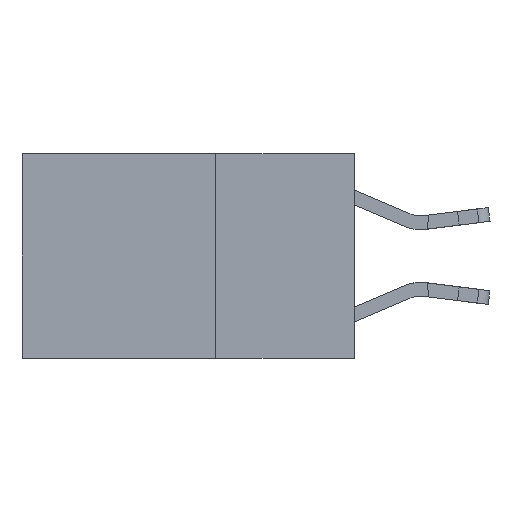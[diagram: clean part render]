
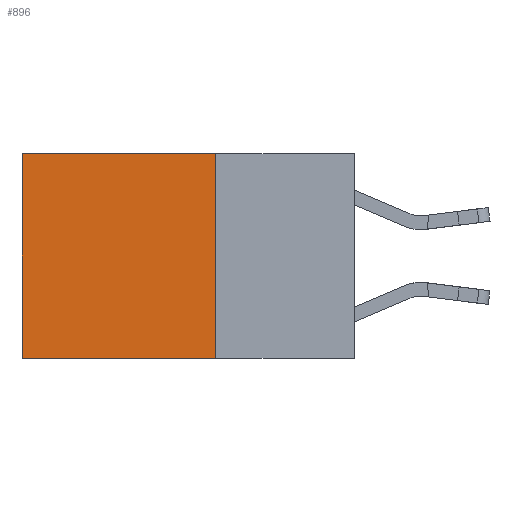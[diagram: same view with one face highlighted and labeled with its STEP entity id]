
A CAD part, left-side view. The second image highlights one B-rep face of the part: STEP entity #896.
In plain terms, the highlighted planar face has unit normal (-1, 0, 0).
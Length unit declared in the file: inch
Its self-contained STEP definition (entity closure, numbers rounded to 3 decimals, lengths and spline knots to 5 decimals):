
#176 = LINE ( 'NONE', #10682, #10564 ) ;
#872 = DIRECTION ( 'NONE',  ( 0., 0., -1. ) ) ;
#896 = ADVANCED_FACE ( 'NONE', ( #1085 ), #10750, .F. ) ;
#969 = VECTOR ( 'NONE', #8218, 39.37008 ) ;
#1085 = FACE_OUTER_BOUND ( 'NONE', #4299, .T. ) ;
#2605 = CARTESIAN_POINT ( 'NONE',  ( 0.2625, 0.6, 0. ) ) ;
#3169 = CARTESIAN_POINT ( 'NONE',  ( 0.2625, 0.25, 0. ) ) ;
#4198 = LINE ( 'NONE', #3169, #969 ) ;
#4299 = EDGE_LOOP ( 'NONE', ( #4817, #12886, #12932, #7563 ) ) ;
#4817 = ORIENTED_EDGE ( 'NONE', *, *, #10227, .T. ) ;
#4929 = EDGE_CURVE ( 'NONE', #14696, #8628, #4198, .T. ) ;
#5153 = VERTEX_POINT ( 'NONE', #7000 ) ;
#5330 = DIRECTION ( 'NONE',  ( 0., 1., 0. ) ) ;
#5485 = VECTOR ( 'NONE', #10080, 39.37008 ) ;
#5500 = LINE ( 'NONE', #12679, #13962 ) ;
#7000 = CARTESIAN_POINT ( 'NONE',  ( 0.2625, 0.6, -0.37 ) ) ;
#7563 = ORIENTED_EDGE ( 'NONE', *, *, #11995, .T. ) ;
#7933 = AXIS2_PLACEMENT_3D ( 'NONE', #8296, #10813, #872 ) ;
#8218 = DIRECTION ( 'NONE',  ( 0., 0., -1. ) ) ;
#8296 = CARTESIAN_POINT ( 'NONE',  ( 0.2625, 0.25, 0. ) ) ;
#8628 = VERTEX_POINT ( 'NONE', #14497 ) ;
#9402 = DIRECTION ( 'NONE',  ( 0., 0., -1. ) ) ;
#10080 = DIRECTION ( 'NONE',  ( 0., 1., 0. ) ) ;
#10227 = EDGE_CURVE ( 'NONE', #12612, #5153, #176, .T. ) ;
#10564 = VECTOR ( 'NONE', #9402, 39.37008 ) ;
#10682 = CARTESIAN_POINT ( 'NONE',  ( 0.2625, 0.6, 0. ) ) ;
#10750 = PLANE ( 'NONE',  #7933 ) ;
#10813 = DIRECTION ( 'NONE',  ( 1., 0., 0. ) ) ;
#11995 = EDGE_CURVE ( 'NONE', #14696, #12612, #14134, .T. ) ;
#12612 = VERTEX_POINT ( 'NONE', #2605 ) ;
#12679 = CARTESIAN_POINT ( 'NONE',  ( 0.2625, 0.25, -0.37 ) ) ;
#12886 = ORIENTED_EDGE ( 'NONE', *, *, #14343, .F. ) ;
#12932 = ORIENTED_EDGE ( 'NONE', *, *, #4929, .F. ) ;
#13962 = VECTOR ( 'NONE', #5330, 39.37008 ) ;
#14134 = LINE ( 'NONE', #14823, #5485 ) ;
#14343 = EDGE_CURVE ( 'NONE', #8628, #5153, #5500, .T. ) ;
#14497 = CARTESIAN_POINT ( 'NONE',  ( 0.2625, 0.25, -0.37 ) ) ;
#14696 = VERTEX_POINT ( 'NONE', #15025 ) ;
#14823 = CARTESIAN_POINT ( 'NONE',  ( 0.2625, 0.25, 0. ) ) ;
#15025 = CARTESIAN_POINT ( 'NONE',  ( 0.2625, 0.25, 0. ) ) ;
